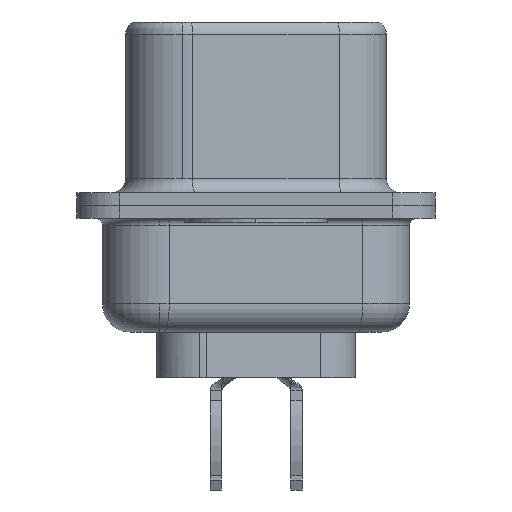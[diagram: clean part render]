
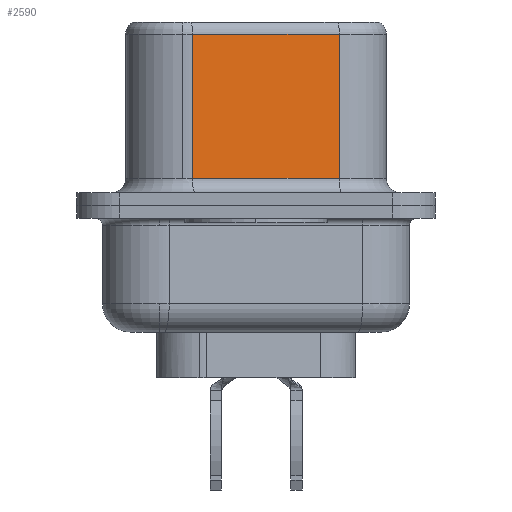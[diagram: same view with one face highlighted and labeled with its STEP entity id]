
A CAD part, left-side view. The second image highlights one B-rep face of the part: STEP entity #2590.
In plain terms, the highlighted planar face has unit normal (-0.985, -0.174, 0).
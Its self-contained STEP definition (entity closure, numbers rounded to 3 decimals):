
#213 = DIRECTION ( 'NONE',  ( 0.985, 0.174, 0. ) ) ;
#308 = CARTESIAN_POINT ( 'NONE',  ( 3.665, 2.233, 6.02 ) ) ;
#1350 = EDGE_CURVE ( 'NONE', #2064, #2304, #8736, .T. ) ;
#1529 = DIRECTION ( 'NONE',  ( -0.174, 0.985, 0. ) ) ;
#2050 = DIRECTION ( 'NONE',  ( 0., 0., -1. ) ) ;
#2064 = VERTEX_POINT ( 'NONE', #8149 ) ;
#2304 = VERTEX_POINT ( 'NONE', #10203 ) ;
#2590 = ADVANCED_FACE ( 'NONE', ( #9820 ), #14492, .F. ) ;
#2990 = VERTEX_POINT ( 'NONE', #4887 ) ;
#3835 = LINE ( 'NONE', #14639, #10073 ) ;
#3857 = EDGE_LOOP ( 'NONE', ( #4840, #11238, #14120, #12602 ) ) ;
#3945 = VECTOR ( 'NONE', #2050, 1000. ) ;
#4411 = CARTESIAN_POINT ( 'NONE',  ( 4.575, -2.927, 6.02 ) ) ;
#4840 = ORIENTED_EDGE ( 'NONE', *, *, #13541, .F. ) ;
#4887 = CARTESIAN_POINT ( 'NONE',  ( 4.575, -2.927, 6.02 ) ) ;
#5216 = DIRECTION ( 'NONE',  ( 0., 0., -1. ) ) ;
#5846 = VECTOR ( 'NONE', #6732, 1000. ) ;
#6732 = DIRECTION ( 'NONE',  ( -0.174, 0.985, 0. ) ) ;
#6840 = LINE ( 'NONE', #12576, #3945 ) ;
#7110 = EDGE_CURVE ( 'NONE', #2990, #12153, #10325, .T. ) ;
#7293 = AXIS2_PLACEMENT_3D ( 'NONE', #8509, #213, #1529 ) ;
#8149 = CARTESIAN_POINT ( 'NONE',  ( 3.665, 2.233, 0.95 ) ) ;
#8199 = VECTOR ( 'NONE', #14489, 1000. ) ;
#8509 = CARTESIAN_POINT ( 'NONE',  ( 4.575, -2.927, 6.52 ) ) ;
#8736 = LINE ( 'NONE', #9969, #8199 ) ;
#9820 = FACE_OUTER_BOUND ( 'NONE', #3857, .T. ) ;
#9969 = CARTESIAN_POINT ( 'NONE',  ( 4.575, -2.927, 0.95 ) ) ;
#10073 = VECTOR ( 'NONE', #5216, 1000. ) ;
#10203 = CARTESIAN_POINT ( 'NONE',  ( 4.575, -2.927, 0.95 ) ) ;
#10325 = LINE ( 'NONE', #4411, #5846 ) ;
#11238 = ORIENTED_EDGE ( 'NONE', *, *, #7110, .T. ) ;
#12153 = VERTEX_POINT ( 'NONE', #308 ) ;
#12576 = CARTESIAN_POINT ( 'NONE',  ( 3.665, 2.233, 6.52 ) ) ;
#12602 = ORIENTED_EDGE ( 'NONE', *, *, #1350, .T. ) ;
#13341 = EDGE_CURVE ( 'NONE', #12153, #2064, #6840, .T. ) ;
#13541 = EDGE_CURVE ( 'NONE', #2990, #2304, #3835, .T. ) ;
#14120 = ORIENTED_EDGE ( 'NONE', *, *, #13341, .T. ) ;
#14489 = DIRECTION ( 'NONE',  ( 0.174, -0.985, 0. ) ) ;
#14492 = PLANE ( 'NONE',  #7293 ) ;
#14639 = CARTESIAN_POINT ( 'NONE',  ( 4.575, -2.927, 6.52 ) ) ;
